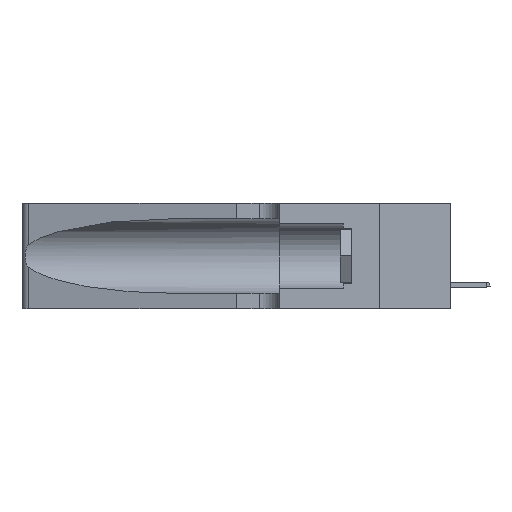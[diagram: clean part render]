
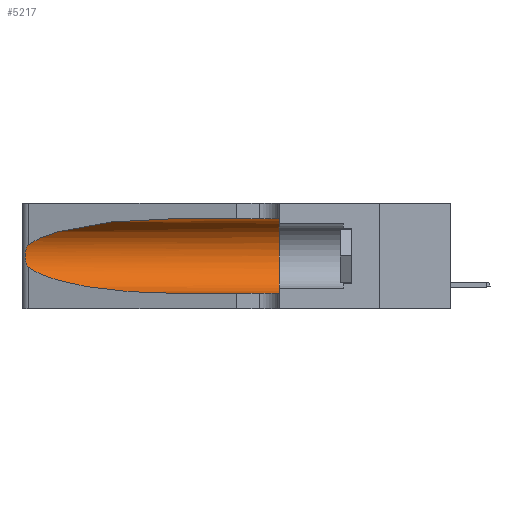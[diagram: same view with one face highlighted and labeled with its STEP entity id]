
A CAD part, left-side view. The second image highlights one B-rep face of the part: STEP entity #5217.
In plain terms, the highlighted cylindrical face has radius 3.308 mm (diameter 6.617 mm), a partial arc.
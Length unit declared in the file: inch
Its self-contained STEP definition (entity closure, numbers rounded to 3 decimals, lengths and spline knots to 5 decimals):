
#136 = LINE ( 'NONE', #4795, #9775 ) ;
#556 = DIRECTION ( 'NONE',  ( 0., -1., 0. ) ) ;
#587 = CARTESIAN_POINT ( 'NONE',  ( 0.26075, 1.23896, 0.19203 ) ) ;
#1421 = ORIENTED_EDGE ( 'NONE', *, *, #38695, .T. ) ;
#4280 = CARTESIAN_POINT ( 'NONE',  ( 0.25487, 1.22718, 0.22369 ) ) ;
#4746 = CARTESIAN_POINT ( 'NONE',  ( 0.25789, 1.23486, 0.15765 ) ) ;
#4795 = CARTESIAN_POINT ( 'NONE',  ( 0.1305, 1.61858, 0.31525 ) ) ;
#5217 = ADVANCED_FACE ( 'NONE', ( #22956 ), #38230, .F. ) ;
#5868 = CARTESIAN_POINT ( 'NONE',  ( 0.2373, 1.15595, 0.28018 ) ) ;
#7726 = CARTESIAN_POINT ( 'NONE',  ( 0.26018, 1.23835, 0.19895 ) ) ;
#7953 = CARTESIAN_POINT ( 'NONE',  ( 0.25555, 1.22993, 0.14849 ) ) ;
#8675 = CARTESIAN_POINT ( 'NONE',  ( 0.1305, 0.72297, 0.05475 ) ) ;
#9775 = VECTOR ( 'NONE', #26725, 39.37008 ) ;
#9884 = CARTESIAN_POINT ( 'NONE',  ( 0.25487, 1.22718, 0.22369 ) ) ;
#9977 = ORIENTED_EDGE ( 'NONE', *, *, #31798, .T. ) ;
#10773 = CARTESIAN_POINT ( 'NONE',  ( 0.1305, 0.35, 0.185 ) ) ;
#12193 = B_SPLINE_CURVE_WITH_KNOTS ( 'NONE', 3,
 ( #4280, #45903, #41481, #41964, #18795, #7726, #587, #22747, #37754, #26681, #4746, #41702, #7953, #22992 ),
 .UNSPECIFIED., .F., .F.,
 ( 4, 2, 2, 2, 2, 2, 4 ),
 ( 0., 0.00027, 0.00053, 0.00107, 0.0016, 0.00187, 0.00214 ),
 .UNSPECIFIED. ) ;
#15063 = CARTESIAN_POINT ( 'NONE',  ( 0.1305, 0.35, 0.31525 ) ) ;
#15752 = VERTEX_POINT ( 'NONE', #24298 ) ;
#16473 = CIRCLE ( 'NONE', #44016, 0.13025 ) ;
#17225 =( BOUNDED_CURVE ( )  B_SPLINE_CURVE ( 3, ( #17677, #25290, #5868, #21123 ),
 .UNSPECIFIED., .F., .F. ) 
 B_SPLINE_CURVE_WITH_KNOTS ( ( 4, 4 ),
 ( 1.5708, 2.84003 ),
 .UNSPECIFIED. ) 
 CURVE ( )  GEOMETRIC_REPRESENTATION_ITEM ( )  RATIONAL_B_SPLINE_CURVE ( ( 1., 0.87, 0.87, 1. ) ) 
 REPRESENTATION_ITEM ( '' )  );
#17644 = DIRECTION ( 'NONE',  ( 0., -1., 0. ) ) ;
#17677 = CARTESIAN_POINT ( 'NONE',  ( 0.1305, 0.72297, 0.31525 ) ) ;
#17861 = EDGE_LOOP ( 'NONE', ( #9977, #28748, #1421, #40232, #40031, #34076 ) ) ;
#18795 = CARTESIAN_POINT ( 'NONE',  ( 0.25854, 1.2359, 0.20912 ) ) ;
#19310 = VERTEX_POINT ( 'NONE', #22295 ) ;
#19995 = AXIS2_PLACEMENT_3D ( 'NONE', #42412, #556, #34298 ) ;
#21123 = CARTESIAN_POINT ( 'NONE',  ( 0.25487, 1.22718, 0.22369 ) ) ;
#22295 = CARTESIAN_POINT ( 'NONE',  ( 0.25487, 1.22718, 0.14631 ) ) ;
#22747 = CARTESIAN_POINT ( 'NONE',  ( 0.26075, 1.23896, 0.178 ) ) ;
#22956 = FACE_OUTER_BOUND ( 'NONE', #17861, .T. ) ;
#22992 = CARTESIAN_POINT ( 'NONE',  ( 0.25487, 1.22718, 0.14631 ) ) ;
#23887 = VERTEX_POINT ( 'NONE', #9884 ) ;
#24298 = CARTESIAN_POINT ( 'NONE',  ( 0.1305, 0.72297, 0.31525 ) ) ;
#25290 = CARTESIAN_POINT ( 'NONE',  ( 0.18966, 0.96281, 0.31525 ) ) ;
#25721 =( BOUNDED_CURVE ( )  B_SPLINE_CURVE ( 3, ( #26677, #46148, #41697, #8675 ),
 .UNSPECIFIED., .F., .T. ) 
 B_SPLINE_CURVE_WITH_KNOTS ( ( 4, 4 ),
 ( 3.44316, 4.71239 ),
 .UNSPECIFIED. ) 
 CURVE ( )  GEOMETRIC_REPRESENTATION_ITEM ( )  RATIONAL_B_SPLINE_CURVE ( ( 1., 0.87, 0.87, 1. ) ) 
 REPRESENTATION_ITEM ( '' )  );
#26677 = CARTESIAN_POINT ( 'NONE',  ( 0.25487, 1.22718, 0.14631 ) ) ;
#26681 = CARTESIAN_POINT ( 'NONE',  ( 0.25856, 1.23593, 0.16098 ) ) ;
#26725 = DIRECTION ( 'NONE',  ( 0., -1., 0. ) ) ;
#28748 = ORIENTED_EDGE ( 'NONE', *, *, #30676, .T. ) ;
#29079 = EDGE_CURVE ( 'NONE', #15752, #40848, #136, .T. ) ;
#30676 = EDGE_CURVE ( 'NONE', #23887, #19310, #12193, .T. ) ;
#31798 = EDGE_CURVE ( 'NONE', #15752, #23887, #17225, .T. ) ;
#31923 = EDGE_CURVE ( 'NONE', #40848, #44524, #16473, .T. ) ;
#33429 = DIRECTION ( 'NONE',  ( 0., 0., 1. ) ) ;
#34076 = ORIENTED_EDGE ( 'NONE', *, *, #29079, .F. ) ;
#34298 = DIRECTION ( 'NONE',  ( 0., 0., -1. ) ) ;
#37754 = CARTESIAN_POINT ( 'NONE',  ( 0.26017, 1.23833, 0.17102 ) ) ;
#38230 = CYLINDRICAL_SURFACE ( 'NONE', #19995, 0.13025 ) ;
#38695 = EDGE_CURVE ( 'NONE', #19310, #44903, #25721, .T. ) ;
#40031 = ORIENTED_EDGE ( 'NONE', *, *, #31923, .F. ) ;
#40232 = ORIENTED_EDGE ( 'NONE', *, *, #41941, .T. ) ;
#40848 = VERTEX_POINT ( 'NONE', #15063 ) ;
#41481 = CARTESIAN_POINT ( 'NONE',  ( 0.25639, 1.23184, 0.21858 ) ) ;
#41544 = DIRECTION ( 'NONE',  ( 0., 1., 0. ) ) ;
#41697 = CARTESIAN_POINT ( 'NONE',  ( 0.18966, 0.96281, 0.05475 ) ) ;
#41702 = CARTESIAN_POINT ( 'NONE',  ( 0.25639, 1.23186, 0.15144 ) ) ;
#41941 = EDGE_CURVE ( 'NONE', #44903, #44524, #46727, .T. ) ;
#41964 = CARTESIAN_POINT ( 'NONE',  ( 0.25787, 1.23484, 0.2124 ) ) ;
#42412 = CARTESIAN_POINT ( 'NONE',  ( 0.1305, 1.61858, 0.185 ) ) ;
#43056 = CARTESIAN_POINT ( 'NONE',  ( 0.1305, 0.35, 0.05475 ) ) ;
#44016 = AXIS2_PLACEMENT_3D ( 'NONE', #10773, #41544, #33429 ) ;
#44178 = CARTESIAN_POINT ( 'NONE',  ( 0.1305, 0.72297, 0.05475 ) ) ;
#44524 = VERTEX_POINT ( 'NONE', #43056 ) ;
#44903 = VERTEX_POINT ( 'NONE', #44178 ) ;
#45382 = VECTOR ( 'NONE', #17644, 39.37008 ) ;
#45903 = CARTESIAN_POINT ( 'NONE',  ( 0.25555, 1.22994, 0.2215 ) ) ;
#46148 = CARTESIAN_POINT ( 'NONE',  ( 0.2373, 1.15595, 0.08982 ) ) ;
#46727 = LINE ( 'NONE', #46969, #45382 ) ;
#46969 = CARTESIAN_POINT ( 'NONE',  ( 0.1305, 1.61858, 0.05475 ) ) ;
